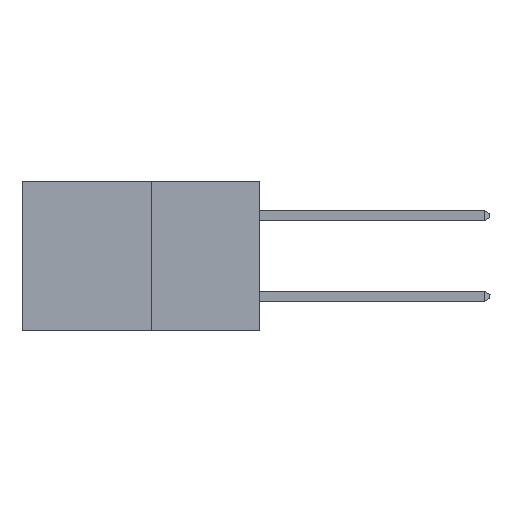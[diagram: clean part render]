
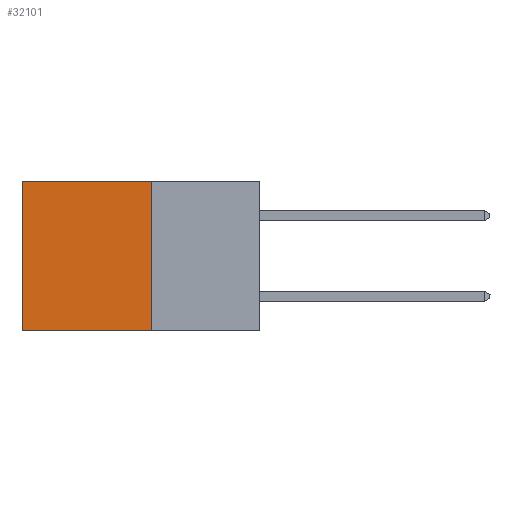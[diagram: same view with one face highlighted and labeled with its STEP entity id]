
A CAD part, left-side view. The second image highlights one B-rep face of the part: STEP entity #32101.
In plain terms, the highlighted planar face has unit normal (-1, 0, 0).
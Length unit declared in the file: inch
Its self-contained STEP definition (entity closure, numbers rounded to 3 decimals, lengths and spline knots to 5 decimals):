
#677 = EDGE_LOOP ( 'NONE', ( #30673, #5287, #25794, #33536 ) ) ;
#2290 = CARTESIAN_POINT ( 'NONE',  ( 0.277, 0.59, -0.37 ) ) ;
#4371 = VECTOR ( 'NONE', #31049, 39.37008 ) ;
#5287 = ORIENTED_EDGE ( 'NONE', *, *, #6222, .F. ) ;
#6222 = EDGE_CURVE ( 'NONE', #21628, #25157, #16786, .T. ) ;
#8765 = EDGE_CURVE ( 'NONE', #20357, #20282, #9750, .T. ) ;
#8804 = CARTESIAN_POINT ( 'NONE',  ( 0.277, 0.27, -0.37 ) ) ;
#9095 = CARTESIAN_POINT ( 'NONE',  ( 0.277, 0.59, -0.37 ) ) ;
#9750 = LINE ( 'NONE', #12540, #22742 ) ;
#9816 = DIRECTION ( 'NONE',  ( 0., 1., 0. ) ) ;
#10242 = CARTESIAN_POINT ( 'NONE',  ( 0.277, 0.27, 0. ) ) ;
#12092 = LINE ( 'NONE', #9095, #31061 ) ;
#12540 = CARTESIAN_POINT ( 'NONE',  ( 0.277, 0.27, 0. ) ) ;
#14461 = DIRECTION ( 'NONE',  ( 1., 0., 0. ) ) ;
#14885 = EDGE_CURVE ( 'NONE', #20357, #21628, #31989, .T. ) ;
#15605 = CARTESIAN_POINT ( 'NONE',  ( 0.277, 0.27, -0.37 ) ) ;
#15967 = VECTOR ( 'NONE', #29080, 39.37008 ) ;
#16680 = CARTESIAN_POINT ( 'NONE',  ( 0.277, 0.27, -0.37 ) ) ;
#16764 = AXIS2_PLACEMENT_3D ( 'NONE', #27284, #14461, #32424 ) ;
#16786 = LINE ( 'NONE', #16680, #15967 ) ;
#20025 = EDGE_CURVE ( 'NONE', #20282, #25157, #12092, .T. ) ;
#20282 = VERTEX_POINT ( 'NONE', #33210 ) ;
#20357 = VERTEX_POINT ( 'NONE', #10242 ) ;
#21628 = VERTEX_POINT ( 'NONE', #8804 ) ;
#22742 = VECTOR ( 'NONE', #9816, 39.37008 ) ;
#24697 = PLANE ( 'NONE',  #16764 ) ;
#25157 = VERTEX_POINT ( 'NONE', #2290 ) ;
#25794 = ORIENTED_EDGE ( 'NONE', *, *, #14885, .F. ) ;
#27284 = CARTESIAN_POINT ( 'NONE',  ( 0.277, 0.27, -0.37 ) ) ;
#28132 = FACE_OUTER_BOUND ( 'NONE', #677, .T. ) ;
#29080 = DIRECTION ( 'NONE',  ( 0., 1., 0. ) ) ;
#29817 = DIRECTION ( 'NONE',  ( 0., 0., -1. ) ) ;
#30673 = ORIENTED_EDGE ( 'NONE', *, *, #20025, .T. ) ;
#31049 = DIRECTION ( 'NONE',  ( 0., 0., -1. ) ) ;
#31061 = VECTOR ( 'NONE', #29817, 39.37008 ) ;
#31989 = LINE ( 'NONE', #15605, #4371 ) ;
#32101 = ADVANCED_FACE ( 'NONE', ( #28132 ), #24697, .F. ) ;
#32424 = DIRECTION ( 'NONE',  ( 0., 0., -1. ) ) ;
#33210 = CARTESIAN_POINT ( 'NONE',  ( 0.277, 0.59, 0. ) ) ;
#33536 = ORIENTED_EDGE ( 'NONE', *, *, #8765, .T. ) ;
